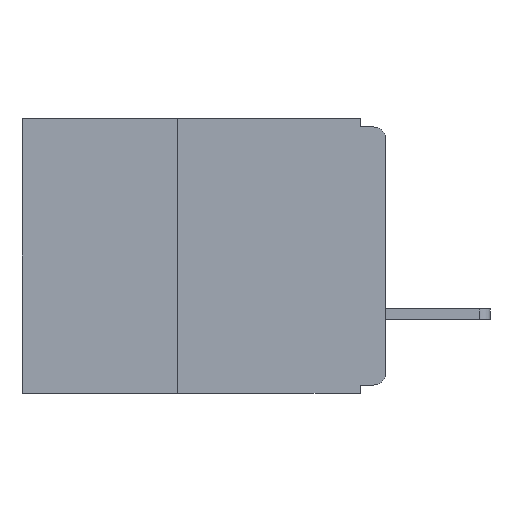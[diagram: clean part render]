
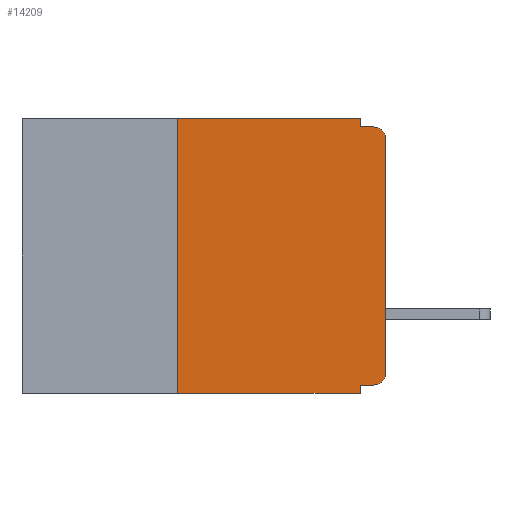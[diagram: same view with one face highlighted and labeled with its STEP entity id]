
A CAD part, left-side view. The second image highlights one B-rep face of the part: STEP entity #14209.
In plain terms, the highlighted planar face has unit normal (-1, 0, 0).
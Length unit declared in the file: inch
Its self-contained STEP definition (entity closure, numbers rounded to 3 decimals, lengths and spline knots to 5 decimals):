
#290 = CARTESIAN_POINT ( 'NONE',  ( 0., 0.031, -0.01 ) ) ;
#389 = CARTESIAN_POINT ( 'NONE',  ( 0., 0.015, -0.305 ) ) ;
#1319 = VERTEX_POINT ( 'NONE', #14583 ) ;
#1752 = CARTESIAN_POINT ( 'NONE',  ( 0., 0.25, -0.33 ) ) ;
#2116 = CARTESIAN_POINT ( 'NONE',  ( 0., 0.015, -0.025 ) ) ;
#2398 = LINE ( 'NONE', #6008, #21022 ) ;
#2660 = VERTEX_POINT ( 'NONE', #7695 ) ;
#2677 = DIRECTION ( 'NONE',  ( 0., 0., -1. ) ) ;
#3522 = VERTEX_POINT ( 'NONE', #290 ) ;
#4094 = LINE ( 'NONE', #14455, #26259 ) ;
#4470 = DIRECTION ( 'NONE',  ( 0., 0., -1. ) ) ;
#4532 = DIRECTION ( 'NONE',  ( 1., 0., 0. ) ) ;
#4645 = EDGE_CURVE ( 'NONE', #25261, #1319, #4094, .T. ) ;
#4771 = AXIS2_PLACEMENT_3D ( 'NONE', #389, #16216, #2677 ) ;
#4848 = ORIENTED_EDGE ( 'NONE', *, *, #25634, .F. ) ;
#5214 = EDGE_LOOP ( 'NONE', ( #12371, #19393, #22433, #23676, #13678, #15725, #8182, #4848, #24227, #18137 ) ) ;
#5883 = CARTESIAN_POINT ( 'NONE',  ( 0., 0., -0.305 ) ) ;
#6008 = CARTESIAN_POINT ( 'NONE',  ( 0., 0.25, -0.33 ) ) ;
#6298 = VECTOR ( 'NONE', #9497, 39.37008 ) ;
#6299 = CARTESIAN_POINT ( 'NONE',  ( 0., 0.25, 0. ) ) ;
#6553 = LINE ( 'NONE', #22974, #11832 ) ;
#6673 = VECTOR ( 'NONE', #8136, 39.37008 ) ;
#6705 = VERTEX_POINT ( 'NONE', #6922 ) ;
#6922 = CARTESIAN_POINT ( 'NONE',  ( 0., 0., -0.025 ) ) ;
#7037 = VERTEX_POINT ( 'NONE', #17066 ) ;
#7166 = CARTESIAN_POINT ( 'NONE',  ( 0., 0.031, 0. ) ) ;
#7547 = DIRECTION ( 'NONE',  ( 0., 0., -1. ) ) ;
#7695 = CARTESIAN_POINT ( 'NONE',  ( 0., 0.015, -0.01 ) ) ;
#7754 = CARTESIAN_POINT ( 'NONE',  ( 0., 0.031, -0.32 ) ) ;
#8136 = DIRECTION ( 'NONE',  ( 0., 0., 1. ) ) ;
#8182 = ORIENTED_EDGE ( 'NONE', *, *, #4645, .T. ) ;
#8383 = LINE ( 'NONE', #22817, #12938 ) ;
#8713 = CARTESIAN_POINT ( 'NONE',  ( 0., 0., -0.32 ) ) ;
#9497 = DIRECTION ( 'NONE',  ( 0., -1., 0. ) ) ;
#9587 = DIRECTION ( 'NONE',  ( 0., 0., -1. ) ) ;
#10383 = CARTESIAN_POINT ( 'NONE',  ( 0., 0., 0. ) ) ;
#11444 = VECTOR ( 'NONE', #7547, 39.37008 ) ;
#11589 = AXIS2_PLACEMENT_3D ( 'NONE', #2116, #17918, #4470 ) ;
#11832 = VECTOR ( 'NONE', #25114, 39.37008 ) ;
#11976 = EDGE_CURVE ( 'NONE', #16028, #3522, #17391, .T. ) ;
#12371 = ORIENTED_EDGE ( 'NONE', *, *, #15782, .T. ) ;
#12938 = VECTOR ( 'NONE', #9587, 39.37008 ) ;
#13520 = CARTESIAN_POINT ( 'NONE',  ( 0., 0.031, 0. ) ) ;
#13678 = ORIENTED_EDGE ( 'NONE', *, *, #24888, .F. ) ;
#13802 = FACE_OUTER_BOUND ( 'NONE', #5214, .T. ) ;
#14209 = ADVANCED_FACE ( 'NONE', ( #13802 ), #26589, .F. ) ;
#14320 = DIRECTION ( 'NONE',  ( 0., -1., 0. ) ) ;
#14455 = CARTESIAN_POINT ( 'NONE',  ( 0., 0.437, -0.33 ) ) ;
#14583 = CARTESIAN_POINT ( 'NONE',  ( 0., 0.031, -0.33 ) ) ;
#14628 = EDGE_CURVE ( 'NONE', #25261, #21654, #2398, .T. ) ;
#15101 = VERTEX_POINT ( 'NONE', #5883 ) ;
#15725 = ORIENTED_EDGE ( 'NONE', *, *, #14628, .F. ) ;
#15782 = EDGE_CURVE ( 'NONE', #15101, #6705, #28649, .T. ) ;
#16028 = VERTEX_POINT ( 'NONE', #13520 ) ;
#16216 = DIRECTION ( 'NONE',  ( -1., 0., 0. ) ) ;
#17066 = CARTESIAN_POINT ( 'NONE',  ( 0., 0.015, -0.32 ) ) ;
#17391 = LINE ( 'NONE', #7166, #11444 ) ;
#17918 = DIRECTION ( 'NONE',  ( -1., 0., 0. ) ) ;
#17983 = CARTESIAN_POINT ( 'NONE',  ( 0., 0.437, 0. ) ) ;
#18037 = CIRCLE ( 'NONE', #4771, 0.015 ) ;
#18137 = ORIENTED_EDGE ( 'NONE', *, *, #27374, .T. ) ;
#19393 = ORIENTED_EDGE ( 'NONE', *, *, #22311, .T. ) ;
#20185 = DIRECTION ( 'NONE',  ( 0., 0., -1. ) ) ;
#20548 = CARTESIAN_POINT ( 'NONE',  ( 0., 0.437, 0. ) ) ;
#21022 = VECTOR ( 'NONE', #21570, 39.37008 ) ;
#21457 = LINE ( 'NONE', #8713, #26506 ) ;
#21570 = DIRECTION ( 'NONE',  ( 0., 0., 1. ) ) ;
#21654 = VERTEX_POINT ( 'NONE', #6299 ) ;
#22311 = EDGE_CURVE ( 'NONE', #6705, #2660, #27514, .T. ) ;
#22433 = ORIENTED_EDGE ( 'NONE', *, *, #26335, .F. ) ;
#22721 = AXIS2_PLACEMENT_3D ( 'NONE', #17983, #4532, #20185 ) ;
#22817 = CARTESIAN_POINT ( 'NONE',  ( 0., 0.031, -0.33 ) ) ;
#22974 = CARTESIAN_POINT ( 'NONE',  ( 0., 0., -0.01 ) ) ;
#23310 = LINE ( 'NONE', #20548, #6298 ) ;
#23676 = ORIENTED_EDGE ( 'NONE', *, *, #11976, .F. ) ;
#24227 = ORIENTED_EDGE ( 'NONE', *, *, #27265, .F. ) ;
#24888 = EDGE_CURVE ( 'NONE', #21654, #16028, #23310, .T. ) ;
#25114 = DIRECTION ( 'NONE',  ( 0., -1., 0. ) ) ;
#25261 = VERTEX_POINT ( 'NONE', #1752 ) ;
#25634 = EDGE_CURVE ( 'NONE', #26446, #1319, #8383, .T. ) ;
#26259 = VECTOR ( 'NONE', #14320, 39.37008 ) ;
#26335 = EDGE_CURVE ( 'NONE', #3522, #2660, #6553, .T. ) ;
#26446 = VERTEX_POINT ( 'NONE', #7754 ) ;
#26506 = VECTOR ( 'NONE', #28410, 39.37008 ) ;
#26589 = PLANE ( 'NONE',  #22721 ) ;
#27265 = EDGE_CURVE ( 'NONE', #7037, #26446, #21457, .T. ) ;
#27374 = EDGE_CURVE ( 'NONE', #7037, #15101, #18037, .T. ) ;
#27514 = CIRCLE ( 'NONE', #11589, 0.015 ) ;
#28410 = DIRECTION ( 'NONE',  ( 0., 1., 0. ) ) ;
#28649 = LINE ( 'NONE', #10383, #6673 ) ;
